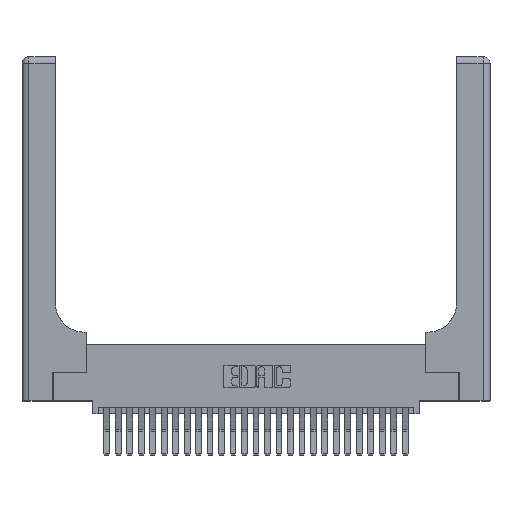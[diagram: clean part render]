
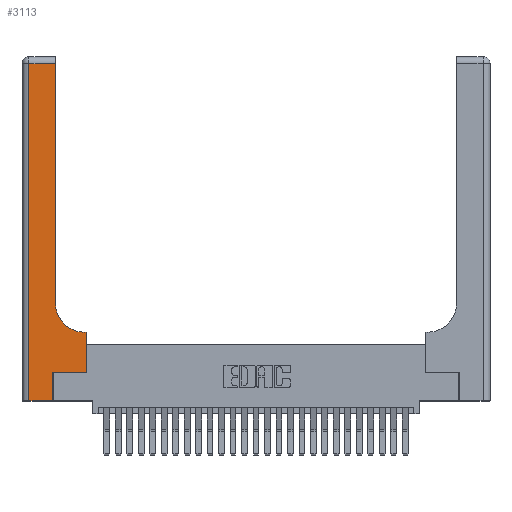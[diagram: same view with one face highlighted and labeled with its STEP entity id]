
A CAD part, top view. The second image highlights one B-rep face of the part: STEP entity #3113.
In plain terms, the highlighted planar face has unit normal (0, 0, 1).
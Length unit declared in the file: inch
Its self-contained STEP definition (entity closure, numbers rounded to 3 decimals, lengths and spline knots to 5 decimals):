
#112 = DIRECTION ( 'NONE',  ( 0., -1., 0. ) ) ;
#698 = CARTESIAN_POINT ( 'NONE',  ( 0., 0., 0.37 ) ) ;
#729 = EDGE_CURVE ( 'NONE', #25531, #9374, #9119, .T. ) ;
#1014 = DIRECTION ( 'NONE',  ( -1., 0., 0. ) ) ;
#1083 = ORIENTED_EDGE ( 'NONE', *, *, #3712, .T. ) ;
#1421 = VERTEX_POINT ( 'NONE', #15398 ) ;
#1905 = DIRECTION ( 'NONE',  ( -1., 0., 0. ) ) ;
#2465 = ORIENTED_EDGE ( 'NONE', *, *, #6826, .T. ) ;
#2606 = DIRECTION ( 'NONE',  ( 0., 1., 0. ) ) ;
#3113 = ADVANCED_FACE ( 'NONE', ( #5236 ), #17050, .F. ) ;
#3292 = DIRECTION ( 'NONE',  ( 0., 1., 0. ) ) ;
#3342 = ORIENTED_EDGE ( 'NONE', *, *, #18870, .T. ) ;
#3712 = EDGE_CURVE ( 'NONE', #1421, #23336, #25420, .T. ) ;
#4872 = CARTESIAN_POINT ( 'NONE',  ( 0.5585, 0.25, 0.37 ) ) ;
#5000 = CARTESIAN_POINT ( 'NONE',  ( 0.2915, 3., 0.37 ) ) ;
#5166 = AXIS2_PLACEMENT_3D ( 'NONE', #21113, #7746, #5725 ) ;
#5236 = FACE_OUTER_BOUND ( 'NONE', #10571, .T. ) ;
#5375 = CARTESIAN_POINT ( 'NONE',  ( 0.5585, 0.6, 0.37 ) ) ;
#5725 = DIRECTION ( 'NONE',  ( 1., 0., 0. ) ) ;
#5740 = CARTESIAN_POINT ( 'NONE',  ( 0.06, 0., 0.37 ) ) ;
#5753 = VERTEX_POINT ( 'NONE', #5375 ) ;
#6826 = EDGE_CURVE ( 'NONE', #9374, #1421, #8291, .T. ) ;
#6854 = CARTESIAN_POINT ( 'NONE',  ( 0.06, 3., 0.37 ) ) ;
#7034 = LINE ( 'NONE', #27786, #15310 ) ;
#7169 = VERTEX_POINT ( 'NONE', #5740 ) ;
#7395 = LINE ( 'NONE', #698, #27111 ) ;
#7592 = CARTESIAN_POINT ( 'NONE',  ( 0.2915, 0.85, 0.37 ) ) ;
#7746 = DIRECTION ( 'NONE',  ( 0., 0., -1. ) ) ;
#8291 = LINE ( 'NONE', #5000, #15855 ) ;
#8424 = EDGE_CURVE ( 'NONE', #11666, #21159, #24124, .T. ) ;
#8524 = VECTOR ( 'NONE', #12569, 39.37008 ) ;
#8898 = CARTESIAN_POINT ( 'NONE',  ( 0., 2.94, 0.37 ) ) ;
#8914 = VECTOR ( 'NONE', #1014, 39.37008 ) ;
#9119 = CIRCLE ( 'NONE', #5166, 0.25 ) ;
#9374 = VERTEX_POINT ( 'NONE', #7592 ) ;
#9382 = DIRECTION ( 'NONE',  ( 1., 0., 0. ) ) ;
#9473 = VECTOR ( 'NONE', #1905, 39.37008 ) ;
#10571 = EDGE_LOOP ( 'NONE', ( #2465, #1083, #22210, #27256, #25274, #18652, #3342, #12741, #13904 ) ) ;
#10862 = EDGE_CURVE ( 'NONE', #5753, #25531, #13080, .T. ) ;
#10956 = DIRECTION ( 'NONE',  ( 1., 0., 0. ) ) ;
#11251 = AXIS2_PLACEMENT_3D ( 'NONE', #25963, #19406, #27888 ) ;
#11666 = VERTEX_POINT ( 'NONE', #20563 ) ;
#11893 = EDGE_CURVE ( 'NONE', #26175, #11666, #17167, .T. ) ;
#12569 = DIRECTION ( 'NONE',  ( 0., 1., 0. ) ) ;
#12741 = ORIENTED_EDGE ( 'NONE', *, *, #10862, .T. ) ;
#13080 = LINE ( 'NONE', #27470, #8914 ) ;
#13811 = CARTESIAN_POINT ( 'NONE',  ( 0.5415, 0.6, 0.37 ) ) ;
#13904 = ORIENTED_EDGE ( 'NONE', *, *, #729, .T. ) ;
#15310 = VECTOR ( 'NONE', #3292, 39.37008 ) ;
#15398 = CARTESIAN_POINT ( 'NONE',  ( 0.2915, 2.94, 0.37 ) ) ;
#15775 = VECTOR ( 'NONE', #10956, 39.37008 ) ;
#15855 = VECTOR ( 'NONE', #2606, 39.37008 ) ;
#17050 = PLANE ( 'NONE',  #11251 ) ;
#17167 = LINE ( 'NONE', #21332, #8524 ) ;
#18363 = EDGE_CURVE ( 'NONE', #7169, #26175, #7395, .T. ) ;
#18652 = ORIENTED_EDGE ( 'NONE', *, *, #8424, .T. ) ;
#18870 = EDGE_CURVE ( 'NONE', #21159, #5753, #7034, .T. ) ;
#19406 = DIRECTION ( 'NONE',  ( 0., 0., -1. ) ) ;
#19754 = EDGE_CURVE ( 'NONE', #23336, #7169, #28478, .T. ) ;
#20181 = CARTESIAN_POINT ( 'NONE',  ( 0.269, 0.25, 0.37 ) ) ;
#20563 = CARTESIAN_POINT ( 'NONE',  ( 0.269, 0.25, 0.37 ) ) ;
#21113 = CARTESIAN_POINT ( 'NONE',  ( 0.5415, 0.85, 0.37 ) ) ;
#21159 = VERTEX_POINT ( 'NONE', #4872 ) ;
#21332 = CARTESIAN_POINT ( 'NONE',  ( 0.269, 0., 0.37 ) ) ;
#21925 = VECTOR ( 'NONE', #112, 39.37008 ) ;
#22210 = ORIENTED_EDGE ( 'NONE', *, *, #19754, .T. ) ;
#22352 = CARTESIAN_POINT ( 'NONE',  ( 0.269, 0., 0.37 ) ) ;
#23336 = VERTEX_POINT ( 'NONE', #25061 ) ;
#24124 = LINE ( 'NONE', #20181, #15775 ) ;
#25061 = CARTESIAN_POINT ( 'NONE',  ( 0.06, 2.94, 0.37 ) ) ;
#25274 = ORIENTED_EDGE ( 'NONE', *, *, #11893, .T. ) ;
#25420 = LINE ( 'NONE', #8898, #9473 ) ;
#25531 = VERTEX_POINT ( 'NONE', #13811 ) ;
#25963 = CARTESIAN_POINT ( 'NONE',  ( 0., 3., 0.37 ) ) ;
#26175 = VERTEX_POINT ( 'NONE', #22352 ) ;
#27111 = VECTOR ( 'NONE', #9382, 39.37008 ) ;
#27256 = ORIENTED_EDGE ( 'NONE', *, *, #18363, .T. ) ;
#27470 = CARTESIAN_POINT ( 'NONE',  ( 0.2915, 0.6, 0.37 ) ) ;
#27786 = CARTESIAN_POINT ( 'NONE',  ( 0.5585, 0.25, 0.37 ) ) ;
#27888 = DIRECTION ( 'NONE',  ( -1., 0., 0. ) ) ;
#28478 = LINE ( 'NONE', #6854, #21925 ) ;
